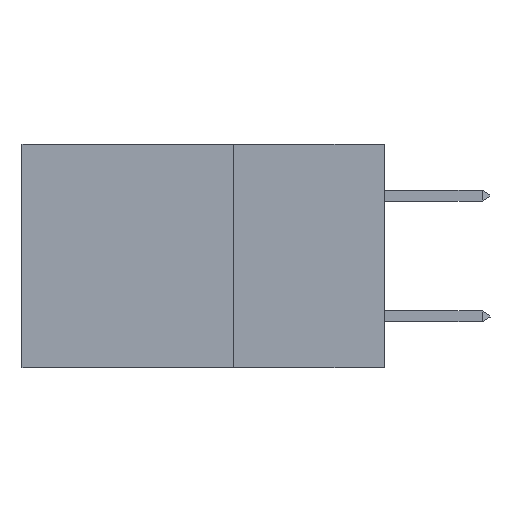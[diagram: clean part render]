
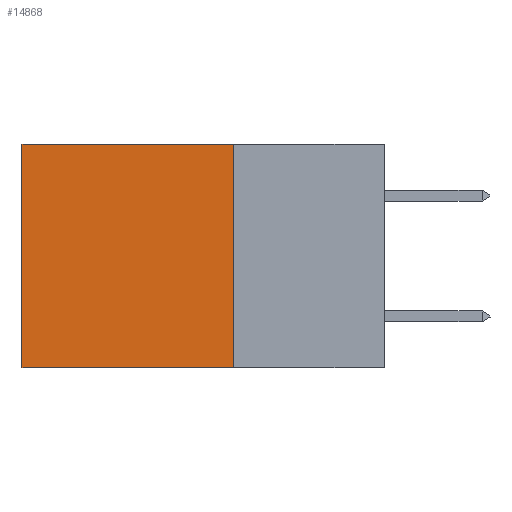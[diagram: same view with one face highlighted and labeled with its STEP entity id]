
A CAD part, left-side view. The second image highlights one B-rep face of the part: STEP entity #14868.
In plain terms, the highlighted planar face has unit normal (-1, 0, 0).
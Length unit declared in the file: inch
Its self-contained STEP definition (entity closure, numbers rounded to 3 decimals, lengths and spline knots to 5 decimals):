
#221 = CARTESIAN_POINT ( 'NONE',  ( 0.2875, 0.25, 0. ) ) ;
#735 = VECTOR ( 'NONE', #26058, 39.37008 ) ;
#1408 = ORIENTED_EDGE ( 'NONE', *, *, #12318, .F. ) ;
#1745 = ORIENTED_EDGE ( 'NONE', *, *, #20614, .F. ) ;
#1888 = DIRECTION ( 'NONE',  ( 1., 0., 0. ) ) ;
#2368 = DIRECTION ( 'NONE',  ( 0., 1., 0. ) ) ;
#3039 = CARTESIAN_POINT ( 'NONE',  ( 0.2875, 0.25, 0. ) ) ;
#5518 = CARTESIAN_POINT ( 'NONE',  ( 0.2875, 0.6, -0.37 ) ) ;
#6399 = VECTOR ( 'NONE', #23545, 39.37008 ) ;
#8043 = CARTESIAN_POINT ( 'NONE',  ( 0.2875, 0.25, 0. ) ) ;
#8253 = CARTESIAN_POINT ( 'NONE',  ( 0.2875, 0.6, 0. ) ) ;
#8779 = VERTEX_POINT ( 'NONE', #5518 ) ;
#8954 = EDGE_LOOP ( 'NONE', ( #14430, #1408, #1745, #25337 ) ) ;
#11582 = VERTEX_POINT ( 'NONE', #14976 ) ;
#11891 = LINE ( 'NONE', #8253, #22118 ) ;
#11896 = LINE ( 'NONE', #3039, #6399 ) ;
#12318 = EDGE_CURVE ( 'NONE', #14880, #8779, #17175, .T. ) ;
#14430 = ORIENTED_EDGE ( 'NONE', *, *, #16709, .T. ) ;
#14819 = LINE ( 'NONE', #221, #24963 ) ;
#14838 = AXIS2_PLACEMENT_3D ( 'NONE', #8043, #1888, #16275 ) ;
#14868 = ADVANCED_FACE ( 'NONE', ( #23458 ), #26302, .F. ) ;
#14880 = VERTEX_POINT ( 'NONE', #26387 ) ;
#14976 = CARTESIAN_POINT ( 'NONE',  ( 0.2875, 0.25, 0. ) ) ;
#15928 = CARTESIAN_POINT ( 'NONE',  ( 0.2875, 0.25, -0.37 ) ) ;
#16053 = CARTESIAN_POINT ( 'NONE',  ( 0.2875, 0.6, 0. ) ) ;
#16275 = DIRECTION ( 'NONE',  ( 0., 0., -1. ) ) ;
#16709 = EDGE_CURVE ( 'NONE', #22464, #8779, #11891, .T. ) ;
#17005 = DIRECTION ( 'NONE',  ( 0., 0., -1. ) ) ;
#17175 = LINE ( 'NONE', #15928, #735 ) ;
#19779 = EDGE_CURVE ( 'NONE', #11582, #22464, #14819, .T. ) ;
#20614 = EDGE_CURVE ( 'NONE', #11582, #14880, #11896, .T. ) ;
#22118 = VECTOR ( 'NONE', #17005, 39.37008 ) ;
#22464 = VERTEX_POINT ( 'NONE', #16053 ) ;
#23458 = FACE_OUTER_BOUND ( 'NONE', #8954, .T. ) ;
#23545 = DIRECTION ( 'NONE',  ( 0., 0., -1. ) ) ;
#24963 = VECTOR ( 'NONE', #2368, 39.37008 ) ;
#25337 = ORIENTED_EDGE ( 'NONE', *, *, #19779, .T. ) ;
#26058 = DIRECTION ( 'NONE',  ( 0., 1., 0. ) ) ;
#26302 = PLANE ( 'NONE',  #14838 ) ;
#26387 = CARTESIAN_POINT ( 'NONE',  ( 0.2875, 0.25, -0.37 ) ) ;
